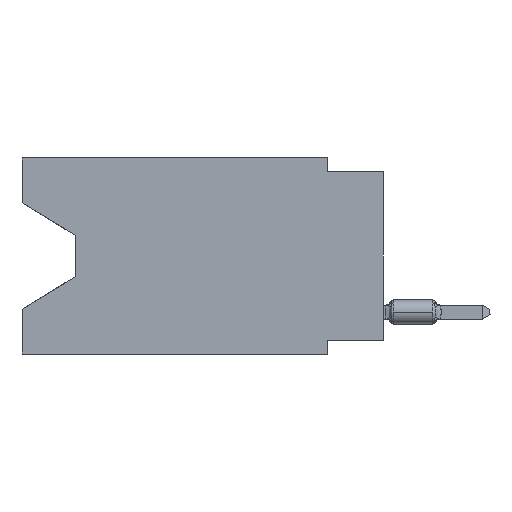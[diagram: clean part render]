
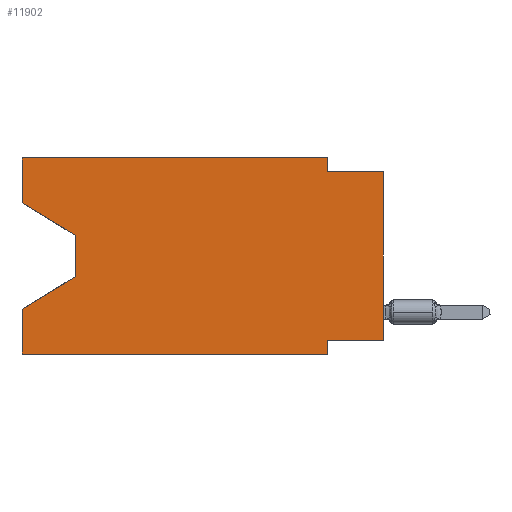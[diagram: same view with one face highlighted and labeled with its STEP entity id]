
A CAD part, left-side view. The second image highlights one B-rep face of the part: STEP entity #11902.
In plain terms, the highlighted planar face has unit normal (-1, 0, 0).
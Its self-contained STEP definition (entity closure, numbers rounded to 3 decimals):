
#382 = LINE ( 'NONE', #10111, #63476 ) ;
#4136 = CARTESIAN_POINT ( 'NONE',  ( 0., 16.383, -8.89 ) ) ;
#4541 = VERTEX_POINT ( 'NONE', #94671 ) ;
#5267 = CARTESIAN_POINT ( 'NONE',  ( 0., 16.383, 0. ) ) ;
#7270 = EDGE_CURVE ( 'NONE', #95008, #17381, #73928, .T. ) ;
#7791 = VERTEX_POINT ( 'NONE', #77309 ) ;
#9244 = EDGE_CURVE ( 'NONE', #55360, #48675, #36786, .T. ) ;
#10111 = CARTESIAN_POINT ( 'NONE',  ( 0., 0., -0.635 ) ) ;
#11902 = ADVANCED_FACE ( 'NONE', ( #72189 ), #78840, .F. ) ;
#11964 = LINE ( 'NONE', #5267, #28402 ) ;
#12251 = ORIENTED_EDGE ( 'NONE', *, *, #7270, .T. ) ;
#13163 = DIRECTION ( 'NONE',  ( 0., 0., -1. ) ) ;
#14406 = DIRECTION ( 'NONE',  ( 0., -0.855, -0.519 ) ) ;
#14892 = DIRECTION ( 'NONE',  ( 0., 1., 0. ) ) ;
#15357 = ORIENTED_EDGE ( 'NONE', *, *, #50483, .F. ) ;
#17381 = VERTEX_POINT ( 'NONE', #21058 ) ;
#17499 = DIRECTION ( 'NONE',  ( 0., 0.855, -0.519 ) ) ;
#17527 = VERTEX_POINT ( 'NONE', #62962 ) ;
#18308 = VECTOR ( 'NONE', #95988, 1000. ) ;
#21050 = DIRECTION ( 'NONE',  ( 0., 0., 1. ) ) ;
#21058 = CARTESIAN_POINT ( 'NONE',  ( 0., 13.97, -5.385 ) ) ;
#21140 = VECTOR ( 'NONE', #42214, 1000. ) ;
#25091 = VECTOR ( 'NONE', #82875, 1000. ) ;
#25563 = CARTESIAN_POINT ( 'NONE',  ( 0., 16.383, 0. ) ) ;
#26201 = CARTESIAN_POINT ( 'NONE',  ( 0., 13.97, -5.385 ) ) ;
#26364 = CARTESIAN_POINT ( 'NONE',  ( 0., 0., 0. ) ) ;
#26732 = VERTEX_POINT ( 'NONE', #82606 ) ;
#27352 = DIRECTION ( 'NONE',  ( 0., 0., -1. ) ) ;
#28402 = VECTOR ( 'NONE', #97904, 1000. ) ;
#28714 = CARTESIAN_POINT ( 'NONE',  ( 0., 16.383, 0. ) ) ;
#28914 = ORIENTED_EDGE ( 'NONE', *, *, #52261, .F. ) ;
#28915 = EDGE_CURVE ( 'NONE', #77287, #4541, #382, .T. ) ;
#29624 = EDGE_CURVE ( 'NONE', #17527, #95008, #54306, .T. ) ;
#30762 = CARTESIAN_POINT ( 'NONE',  ( 0., 16.383, -2.038 ) ) ;
#30914 = EDGE_CURVE ( 'NONE', #17381, #61082, #66119, .T. ) ;
#31414 = VECTOR ( 'NONE', #17499, 1000. ) ;
#32363 = EDGE_CURVE ( 'NONE', #17527, #51148, #98789, .T. ) ;
#32828 = VECTOR ( 'NONE', #14406, 1000. ) ;
#36786 = LINE ( 'NONE', #58336, #25091 ) ;
#39602 = ORIENTED_EDGE ( 'NONE', *, *, #32363, .F. ) ;
#40942 = EDGE_CURVE ( 'NONE', #26732, #48675, #97324, .T. ) ;
#42214 = DIRECTION ( 'NONE',  ( 0., 0., 1. ) ) ;
#42397 = ORIENTED_EDGE ( 'NONE', *, *, #76353, .T. ) ;
#42784 = CARTESIAN_POINT ( 'NONE',  ( 0., 16.383, 0. ) ) ;
#45609 = CARTESIAN_POINT ( 'NONE',  ( 0., 0., -8.255 ) ) ;
#48067 = AXIS2_PLACEMENT_3D ( 'NONE', #49143, #64504, #72699 ) ;
#48675 = VERTEX_POINT ( 'NONE', #56076 ) ;
#48682 = ORIENTED_EDGE ( 'NONE', *, *, #29624, .T. ) ;
#49143 = CARTESIAN_POINT ( 'NONE',  ( 0., 16.383, 0. ) ) ;
#49749 = ORIENTED_EDGE ( 'NONE', *, *, #40942, .F. ) ;
#50483 = EDGE_CURVE ( 'NONE', #51148, #58380, #71986, .T. ) ;
#51148 = VERTEX_POINT ( 'NONE', #25563 ) ;
#52261 = EDGE_CURVE ( 'NONE', #55360, #61082, #11964, .T. ) ;
#54286 = LINE ( 'NONE', #45609, #80997 ) ;
#54306 = LINE ( 'NONE', #30762, #32828 ) ;
#55360 = VERTEX_POINT ( 'NONE', #4136 ) ;
#55458 = CARTESIAN_POINT ( 'NONE',  ( 0., 2.54, 0. ) ) ;
#56076 = CARTESIAN_POINT ( 'NONE',  ( 0., 2.54, -8.89 ) ) ;
#57678 = EDGE_LOOP ( 'NONE', ( #48682, #12251, #93763, #28914, #65960, #49749, #78186, #42397, #86877, #84996, #15357, #39602 ) ) ;
#58336 = CARTESIAN_POINT ( 'NONE',  ( 0., 16.383, -8.89 ) ) ;
#58380 = VERTEX_POINT ( 'NONE', #55458 ) ;
#60859 = CARTESIAN_POINT ( 'NONE',  ( 0., 16.383, -6.852 ) ) ;
#61082 = VERTEX_POINT ( 'NONE', #60859 ) ;
#61257 = LINE ( 'NONE', #69447, #61409 ) ;
#61409 = VECTOR ( 'NONE', #13163, 1000. ) ;
#61534 = VECTOR ( 'NONE', #97828, 1000. ) ;
#62962 = CARTESIAN_POINT ( 'NONE',  ( 0., 16.383, -2.038 ) ) ;
#63476 = VECTOR ( 'NONE', #86887, 1000. ) ;
#63761 = CARTESIAN_POINT ( 'NONE',  ( 0., 2.54, -0.635 ) ) ;
#64504 = DIRECTION ( 'NONE',  ( 1., 0., 0. ) ) ;
#65960 = ORIENTED_EDGE ( 'NONE', *, *, #9244, .T. ) ;
#66119 = LINE ( 'NONE', #26201, #31414 ) ;
#66246 = CARTESIAN_POINT ( 'NONE',  ( 0., 13.97, -3.505 ) ) ;
#67156 = CARTESIAN_POINT ( 'NONE',  ( 0., 2.54, -8.89 ) ) ;
#69447 = CARTESIAN_POINT ( 'NONE',  ( 0., 2.54, 0. ) ) ;
#70768 = EDGE_CURVE ( 'NONE', #58380, #77287, #61257, .T. ) ;
#71986 = LINE ( 'NONE', #42784, #18308 ) ;
#72189 = FACE_OUTER_BOUND ( 'NONE', #57678, .T. ) ;
#72699 = DIRECTION ( 'NONE',  ( 0., 0., -1. ) ) ;
#73928 = LINE ( 'NONE', #66246, #83743 ) ;
#76353 = EDGE_CURVE ( 'NONE', #7791, #4541, #94401, .T. ) ;
#77287 = VERTEX_POINT ( 'NONE', #63761 ) ;
#77309 = CARTESIAN_POINT ( 'NONE',  ( 0., 0., -8.255 ) ) ;
#78186 = ORIENTED_EDGE ( 'NONE', *, *, #99262, .F. ) ;
#78840 = PLANE ( 'NONE',  #48067 ) ;
#80680 = VECTOR ( 'NONE', #21050, 1000. ) ;
#80997 = VECTOR ( 'NONE', #14892, 1000. ) ;
#82606 = CARTESIAN_POINT ( 'NONE',  ( 0., 2.54, -8.255 ) ) ;
#82875 = DIRECTION ( 'NONE',  ( 0., -1., 0. ) ) ;
#83743 = VECTOR ( 'NONE', #27352, 1000. ) ;
#84996 = ORIENTED_EDGE ( 'NONE', *, *, #70768, .F. ) ;
#86877 = ORIENTED_EDGE ( 'NONE', *, *, #28915, .F. ) ;
#86887 = DIRECTION ( 'NONE',  ( 0., -1., 0. ) ) ;
#90690 = CARTESIAN_POINT ( 'NONE',  ( 0., 13.97, -3.505 ) ) ;
#93763 = ORIENTED_EDGE ( 'NONE', *, *, #30914, .T. ) ;
#94401 = LINE ( 'NONE', #26364, #21140 ) ;
#94671 = CARTESIAN_POINT ( 'NONE',  ( 0., 0., -0.635 ) ) ;
#95008 = VERTEX_POINT ( 'NONE', #90690 ) ;
#95988 = DIRECTION ( 'NONE',  ( 0., -1., 0. ) ) ;
#97324 = LINE ( 'NONE', #67156, #61534 ) ;
#97828 = DIRECTION ( 'NONE',  ( 0., 0., -1. ) ) ;
#97904 = DIRECTION ( 'NONE',  ( 0., 0., 1. ) ) ;
#98789 = LINE ( 'NONE', #28714, #80680 ) ;
#99262 = EDGE_CURVE ( 'NONE', #7791, #26732, #54286, .T. ) ;
